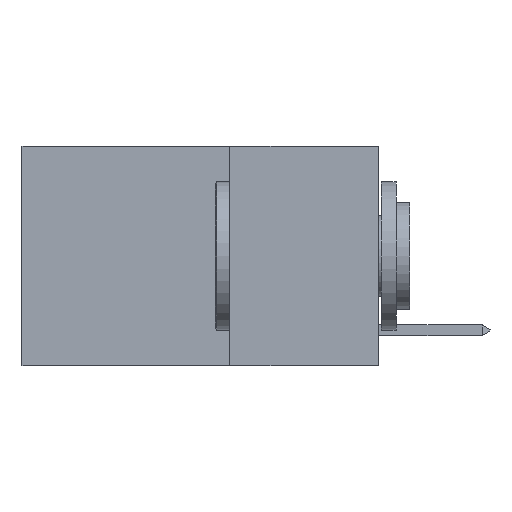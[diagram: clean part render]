
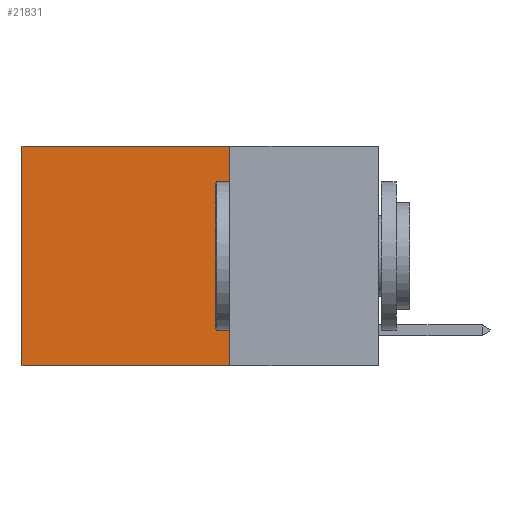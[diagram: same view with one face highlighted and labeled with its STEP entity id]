
A CAD part, left-side view. The second image highlights one B-rep face of the part: STEP entity #21831.
In plain terms, the highlighted planar face has unit normal (-1, 0, 0).
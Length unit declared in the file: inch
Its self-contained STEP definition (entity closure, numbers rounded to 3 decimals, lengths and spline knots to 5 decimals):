
#381 = LINE ( 'NONE', #23932, #18041 ) ;
#387 = FACE_OUTER_BOUND ( 'NONE', #4777, .T. ) ;
#1595 = EDGE_CURVE ( 'NONE', #15789, #12024, #381, .T. ) ;
#2210 = DIRECTION ( 'NONE',  ( 0., 0., -1. ) ) ;
#3224 = VERTEX_POINT ( 'NONE', #11687 ) ;
#4097 = CARTESIAN_POINT ( 'NONE',  ( 0.2625, 0.25, 0. ) ) ;
#4777 = EDGE_LOOP ( 'NONE', ( #20143, #21188, #23631, #9757 ) ) ;
#4786 = VECTOR ( 'NONE', #9045, 39.37008 ) ;
#4985 = EDGE_CURVE ( 'NONE', #3224, #19205, #9857, .T. ) ;
#5534 = DIRECTION ( 'NONE',  ( 0., 1., 0. ) ) ;
#5608 = CARTESIAN_POINT ( 'NONE',  ( 0.2625, 0.6, 0. ) ) ;
#5845 = CARTESIAN_POINT ( 'NONE',  ( 0.2625, 0.25, 0. ) ) ;
#6475 = DIRECTION ( 'NONE',  ( 0., 0., -1. ) ) ;
#7639 = CARTESIAN_POINT ( 'NONE',  ( 0.2625, 0.6, -0.37 ) ) ;
#8039 = DIRECTION ( 'NONE',  ( 0., 0., -1. ) ) ;
#9045 = DIRECTION ( 'NONE',  ( 0., 1., 0. ) ) ;
#9311 = VECTOR ( 'NONE', #2210, 39.37008 ) ;
#9491 = CARTESIAN_POINT ( 'NONE',  ( 0.2625, 0.25, 0. ) ) ;
#9757 = ORIENTED_EDGE ( 'NONE', *, *, #10748, .T. ) ;
#9857 = LINE ( 'NONE', #4097, #9311 ) ;
#10331 = VECTOR ( 'NONE', #5534, 39.37008 ) ;
#10748 = EDGE_CURVE ( 'NONE', #3224, #15789, #16976, .T. ) ;
#11184 = EDGE_CURVE ( 'NONE', #19205, #12024, #13755, .T. ) ;
#11687 = CARTESIAN_POINT ( 'NONE',  ( 0.2625, 0.25, 0. ) ) ;
#12024 = VERTEX_POINT ( 'NONE', #7639 ) ;
#13755 = LINE ( 'NONE', #18248, #4786 ) ;
#15512 = DIRECTION ( 'NONE',  ( 1., 0., 0. ) ) ;
#15539 = CARTESIAN_POINT ( 'NONE',  ( 0.2625, 0.25, -0.37 ) ) ;
#15789 = VERTEX_POINT ( 'NONE', #5608 ) ;
#16976 = LINE ( 'NONE', #5845, #10331 ) ;
#18041 = VECTOR ( 'NONE', #6475, 39.37008 ) ;
#18248 = CARTESIAN_POINT ( 'NONE',  ( 0.2625, 0.25, -0.37 ) ) ;
#18273 = AXIS2_PLACEMENT_3D ( 'NONE', #9491, #15512, #8039 ) ;
#19205 = VERTEX_POINT ( 'NONE', #15539 ) ;
#19230 = PLANE ( 'NONE',  #18273 ) ;
#20143 = ORIENTED_EDGE ( 'NONE', *, *, #1595, .T. ) ;
#21188 = ORIENTED_EDGE ( 'NONE', *, *, #11184, .F. ) ;
#21831 = ADVANCED_FACE ( 'NONE', ( #387 ), #19230, .F. ) ;
#23631 = ORIENTED_EDGE ( 'NONE', *, *, #4985, .F. ) ;
#23932 = CARTESIAN_POINT ( 'NONE',  ( 0.2625, 0.6, 0. ) ) ;
